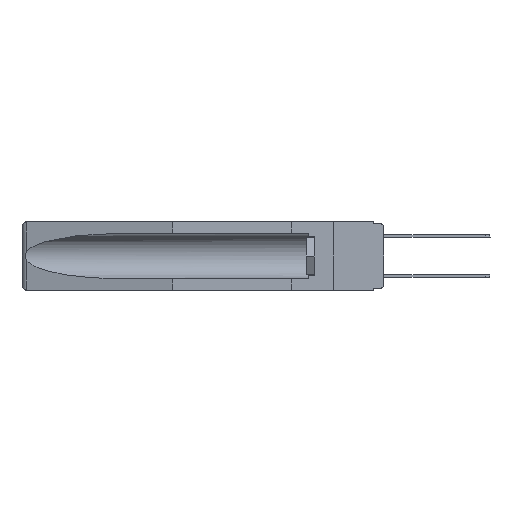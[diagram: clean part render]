
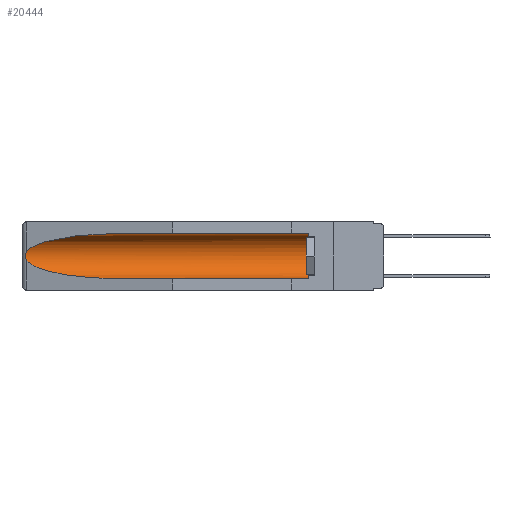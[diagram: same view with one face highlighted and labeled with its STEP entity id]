
A CAD part, left-side view. The second image highlights one B-rep face of the part: STEP entity #20444.
In plain terms, the highlighted cylindrical face has radius 2.857 mm (diameter 5.715 mm), a partial arc.
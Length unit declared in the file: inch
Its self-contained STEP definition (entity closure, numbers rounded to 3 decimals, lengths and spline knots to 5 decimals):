
#830 = DIRECTION ( 'NONE',  ( 0., 0., 1. ) ) ;
#952 = CARTESIAN_POINT ( 'NONE',  ( 0.155, 1.07973, -0.059 ) ) ;
#1077 = DIRECTION ( 'NONE',  ( 0., -1., 0. ) ) ;
#1413 = VERTEX_POINT ( 'NONE', #3013 ) ;
#1536 = CARTESIAN_POINT ( 'NONE',  ( 0.155, 0.126, -0.059 ) ) ;
#1665 = CARTESIAN_POINT ( 'NONE',  ( 0.155, -0.30754, -0.059 ) ) ;
#1735 = CARTESIAN_POINT ( 'NONE',  ( 0.26537, 1.52718, -0.14972 ) ) ;
#1922 = DIRECTION ( 'NONE',  ( 0., 1., 0. ) ) ;
#1992 = CARTESIAN_POINT ( 'NONE',  ( 0.26654, 1.53092, -0.15636 ) ) ;
#2275 = FACE_OUTER_BOUND ( 'NONE', #9214, .T. ) ;
#3013 = CARTESIAN_POINT ( 'NONE',  ( 0.26537, 1.52718, -0.14972 ) ) ;
#4075 = CYLINDRICAL_SURFACE ( 'NONE', #24667, 0.1125 ) ;
#4675 = CARTESIAN_POINT ( 'NONE',  ( 0.26537, 1.52718, -0.14972 ) ) ;
#5345 = ORIENTED_EDGE ( 'NONE', *, *, #10234, .F. ) ;
#5597 = EDGE_CURVE ( 'NONE', #21085, #20781, #11102, .T. ) ;
#5729 =( BOUNDED_CURVE ( )  B_SPLINE_CURVE ( 3, ( #22618, #9165, #21596, #17748 ),
 .UNSPECIFIED., .F., .F. ) 
 B_SPLINE_CURVE_WITH_KNOTS ( ( 4, 4 ),
 ( 0.1948, 1.5708 ),
 .UNSPECIFIED. ) 
 CURVE ( )  GEOMETRIC_REPRESENTATION_ITEM ( )  RATIONAL_B_SPLINE_CURVE ( ( 1., 0.848, 0.848, 1. ) ) 
 REPRESENTATION_ITEM ( '' )  );
#5962 = EDGE_CURVE ( 'NONE', #20781, #1413, #23201, .T. ) ;
#6184 = LINE ( 'NONE', #13952, #9216 ) ;
#6466 = CARTESIAN_POINT ( 'NONE',  ( 0.155, 1.07973, -0.059 ) ) ;
#6650 = VERTEX_POINT ( 'NONE', #17030 ) ;
#7594 = DIRECTION ( 'NONE',  ( 0., 0., 1. ) ) ;
#7840 = CARTESIAN_POINT ( 'NONE',  ( 0.2673, 1.5327, -0.16383 ) ) ;
#7879 = ORIENTED_EDGE ( 'NONE', *, *, #5597, .T. ) ;
#7986 = ORIENTED_EDGE ( 'NONE', *, *, #18976, .T. ) ;
#9165 = CARTESIAN_POINT ( 'NONE',  ( 0.25451, 1.48313, -0.24835 ) ) ;
#9214 = EDGE_LOOP ( 'NONE', ( #21098, #20525, #21147, #5345, #7986, #7879 ) ) ;
#9216 = VECTOR ( 'NONE', #23457, 39.37008 ) ;
#9773 = CARTESIAN_POINT ( 'NONE',  ( 0.2675, 1.53308, -0.17534 ) ) ;
#10234 = EDGE_CURVE ( 'NONE', #15712, #19832, #6184, .T. ) ;
#10620 = CARTESIAN_POINT ( 'NONE',  ( 0.25451, 1.48313, -0.09465 ) ) ;
#10820 = EDGE_CURVE ( 'NONE', #6650, #19832, #5729, .T. ) ;
#11102 = LINE ( 'NONE', #1665, #17795 ) ;
#12419 = CARTESIAN_POINT ( 'NONE',  ( 0.21114, 1.30732, -0.059 ) ) ;
#13262 = CARTESIAN_POINT ( 'NONE',  ( 0.155, 0.126, -0.284 ) ) ;
#13371 = DIRECTION ( 'NONE',  ( 0., 1., 0. ) ) ;
#13952 = CARTESIAN_POINT ( 'NONE',  ( 0.155, -0.30754, -0.284 ) ) ;
#14467 = AXIS2_PLACEMENT_3D ( 'NONE', #24233, #1077, #830 ) ;
#15492 = CARTESIAN_POINT ( 'NONE',  ( 0.155, -0.30754, -0.1715 ) ) ;
#15712 = VERTEX_POINT ( 'NONE', #13262 ) ;
#17030 = CARTESIAN_POINT ( 'NONE',  ( 0.26537, 1.52718, -0.19328 ) ) ;
#17358 = CARTESIAN_POINT ( 'NONE',  ( 0.26597, 1.52961, -0.15275 ) ) ;
#17443 = CARTESIAN_POINT ( 'NONE',  ( 0.26537, 1.52718, -0.19328 ) ) ;
#17748 = CARTESIAN_POINT ( 'NONE',  ( 0.155, 1.07973, -0.284 ) ) ;
#17795 = VECTOR ( 'NONE', #13371, 39.37008 ) ;
#17910 = B_SPLINE_CURVE_WITH_KNOTS ( 'NONE', 3,
 ( #1735, #17358, #1992, #7840, #25129, #9773, #23256, #25219, #23429, #17443 ),
 .UNSPECIFIED., .F., .F.,
 ( 4, 2, 2, 2, 4 ),
 ( 0., 0.00029, 0.00058, 0.00087, 0.00117 ),
 .UNSPECIFIED. ) ;
#18820 = CARTESIAN_POINT ( 'NONE',  ( 0.155, 1.07973, -0.284 ) ) ;
#18976 = EDGE_CURVE ( 'NONE', #15712, #21085, #21232, .T. ) ;
#19832 = VERTEX_POINT ( 'NONE', #18820 ) ;
#19892 = EDGE_CURVE ( 'NONE', #1413, #6650, #17910, .T. ) ;
#20444 = ADVANCED_FACE ( 'NONE', ( #2275 ), #4075, .F. ) ;
#20525 = ORIENTED_EDGE ( 'NONE', *, *, #19892, .T. ) ;
#20781 = VERTEX_POINT ( 'NONE', #6466 ) ;
#21085 = VERTEX_POINT ( 'NONE', #1536 ) ;
#21098 = ORIENTED_EDGE ( 'NONE', *, *, #5962, .T. ) ;
#21147 = ORIENTED_EDGE ( 'NONE', *, *, #10820, .T. ) ;
#21232 = CIRCLE ( 'NONE', #14467, 0.1125 ) ;
#21596 = CARTESIAN_POINT ( 'NONE',  ( 0.21114, 1.30732, -0.284 ) ) ;
#22618 = CARTESIAN_POINT ( 'NONE',  ( 0.26537, 1.52718, -0.19328 ) ) ;
#23201 =( BOUNDED_CURVE ( )  B_SPLINE_CURVE ( 3, ( #952, #12419, #10620, #4675 ),
 .UNSPECIFIED., .F., .T. ) 
 B_SPLINE_CURVE_WITH_KNOTS ( ( 4, 4 ),
 ( 4.71239, 6.08839 ),
 .UNSPECIFIED. ) 
 CURVE ( )  GEOMETRIC_REPRESENTATION_ITEM ( )  RATIONAL_B_SPLINE_CURVE ( ( 1., 0.848, 0.848, 1. ) ) 
 REPRESENTATION_ITEM ( '' )  );
#23256 = CARTESIAN_POINT ( 'NONE',  ( 0.2673, 1.53269, -0.17917 ) ) ;
#23429 = CARTESIAN_POINT ( 'NONE',  ( 0.26597, 1.5296, -0.19026 ) ) ;
#23457 = DIRECTION ( 'NONE',  ( 0., 1., 0. ) ) ;
#24233 = CARTESIAN_POINT ( 'NONE',  ( 0.155, 0.126, -0.1715 ) ) ;
#24667 = AXIS2_PLACEMENT_3D ( 'NONE', #15492, #1922, #7594 ) ;
#25129 = CARTESIAN_POINT ( 'NONE',  ( 0.2675, 1.53308, -0.16763 ) ) ;
#25219 = CARTESIAN_POINT ( 'NONE',  ( 0.26655, 1.53094, -0.18657 ) ) ;
